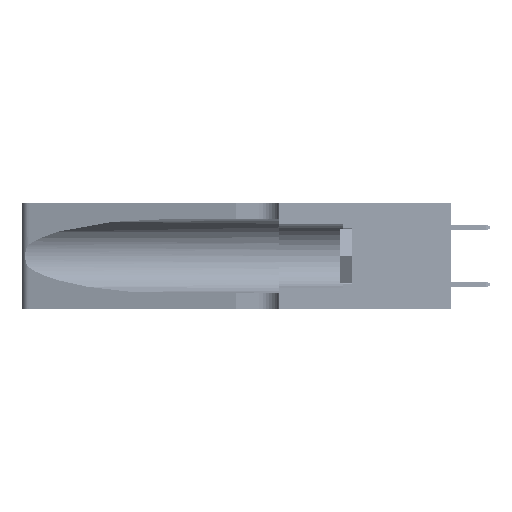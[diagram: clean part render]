
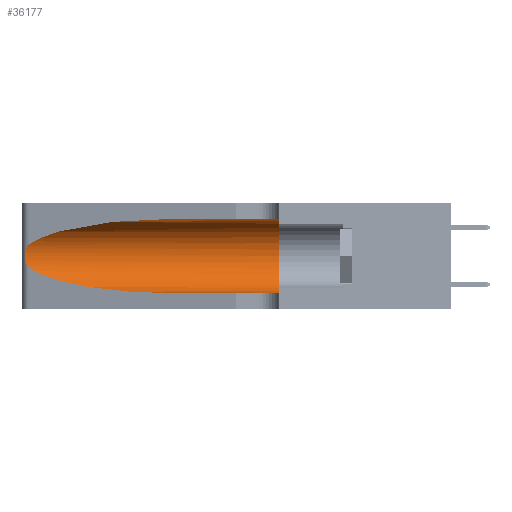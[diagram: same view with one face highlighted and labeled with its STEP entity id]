
A CAD part, left-side view. The second image highlights one B-rep face of the part: STEP entity #36177.
In plain terms, the highlighted cylindrical face has radius 3.308 mm (diameter 6.617 mm), a partial arc.
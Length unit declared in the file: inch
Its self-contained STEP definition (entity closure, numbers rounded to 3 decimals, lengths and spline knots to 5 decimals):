
#191 = VECTOR ( 'NONE', #29480, 39.37008 ) ;
#1337 = ORIENTED_EDGE ( 'NONE', *, *, #4520, .T. ) ;
#3465 = ORIENTED_EDGE ( 'NONE', *, *, #43835, .F. ) ;
#3618 = DIRECTION ( 'NONE',  ( 0., -1., 0. ) ) ;
#4151 = CARTESIAN_POINT ( 'NONE',  ( 0.25854, 1.2359, 0.20912 ) ) ;
#4520 = EDGE_CURVE ( 'NONE', #49002, #5500, #7059, .T. ) ;
#4654 = CARTESIAN_POINT ( 'NONE',  ( 0.25487, 1.22718, 0.22369 ) ) ;
#5500 = VERTEX_POINT ( 'NONE', #46580 ) ;
#6939 = CARTESIAN_POINT ( 'NONE',  ( 0.25555, 1.22994, 0.2215 ) ) ;
#7038 = VERTEX_POINT ( 'NONE', #29542 ) ;
#7059 = B_SPLINE_CURVE_WITH_KNOTS ( 'NONE', 3,
 ( #38008, #6939, #23204, #18938, #4151, #26720, #15172, #26460, #30473, #42260, #7921, #11437, #42010, #7432 ),
 .UNSPECIFIED., .F., .F.,
 ( 4, 2, 2, 2, 2, 2, 4 ),
 ( 0., 0.00027, 0.00053, 0.00107, 0.0016, 0.00187, 0.00214 ),
 .UNSPECIFIED. ) ;
#7432 = CARTESIAN_POINT ( 'NONE',  ( 0.25487, 1.22718, 0.14631 ) ) ;
#7582 = FACE_OUTER_BOUND ( 'NONE', #7714, .T. ) ;
#7714 = EDGE_LOOP ( 'NONE', ( #15590, #1337, #43993, #9065, #46394, #3465 ) ) ;
#7921 = CARTESIAN_POINT ( 'NONE',  ( 0.25789, 1.23486, 0.15765 ) ) ;
#8184 = CARTESIAN_POINT ( 'NONE',  ( 0.1305, 0.72297, 0.31525 ) ) ;
#9062 = CARTESIAN_POINT ( 'NONE',  ( 0.1305, 1.61858, 0.185 ) ) ;
#9065 = ORIENTED_EDGE ( 'NONE', *, *, #48445, .T. ) ;
#10133 = CIRCLE ( 'NONE', #30968, 0.13025 ) ;
#10639 = LINE ( 'NONE', #29927, #42033 ) ;
#11437 = CARTESIAN_POINT ( 'NONE',  ( 0.25639, 1.23186, 0.15144 ) ) ;
#15172 = CARTESIAN_POINT ( 'NONE',  ( 0.26075, 1.23896, 0.19203 ) ) ;
#15590 = ORIENTED_EDGE ( 'NONE', *, *, #33847, .T. ) ;
#18763 = CARTESIAN_POINT ( 'NONE',  ( 0.25487, 1.22718, 0.14631 ) ) ;
#18938 = CARTESIAN_POINT ( 'NONE',  ( 0.25787, 1.23484, 0.2124 ) ) ;
#19175 =( BOUNDED_CURVE ( )  B_SPLINE_CURVE ( 3, ( #8184, #23458, #41339, #4654 ),
 .UNSPECIFIED., .F., .T. ) 
 B_SPLINE_CURVE_WITH_KNOTS ( ( 4, 4 ),
 ( 1.5708, 2.84003 ),
 .UNSPECIFIED. ) 
 CURVE ( )  GEOMETRIC_REPRESENTATION_ITEM ( )  RATIONAL_B_SPLINE_CURVE ( ( 1., 0.87, 0.87, 1. ) ) 
 REPRESENTATION_ITEM ( '' )  );
#19764 = CARTESIAN_POINT ( 'NONE',  ( 0.1305, 0.72297, 0.05475 ) ) ;
#19955 = DIRECTION ( 'NONE',  ( 0., 1., 0. ) ) ;
#20069 = CYLINDRICAL_SURFACE ( 'NONE', #26952, 0.13025 ) ;
#20295 = VERTEX_POINT ( 'NONE', #32686 ) ;
#22842 = EDGE_CURVE ( 'NONE', #7038, #20295, #10133, .T. ) ;
#23204 = CARTESIAN_POINT ( 'NONE',  ( 0.25639, 1.23184, 0.21858 ) ) ;
#23458 = CARTESIAN_POINT ( 'NONE',  ( 0.18966, 0.96281, 0.31525 ) ) ;
#24816 = DIRECTION ( 'NONE',  ( 0., 0., -1. ) ) ;
#25413 = VERTEX_POINT ( 'NONE', #19764 ) ;
#26460 = CARTESIAN_POINT ( 'NONE',  ( 0.26075, 1.23896, 0.178 ) ) ;
#26720 = CARTESIAN_POINT ( 'NONE',  ( 0.26018, 1.23835, 0.19895 ) ) ;
#26952 = AXIS2_PLACEMENT_3D ( 'NONE', #9062, #31623, #24816 ) ;
#29480 = DIRECTION ( 'NONE',  ( 0., -1., 0. ) ) ;
#29542 = CARTESIAN_POINT ( 'NONE',  ( 0.1305, 0.35, 0.31525 ) ) ;
#29927 = CARTESIAN_POINT ( 'NONE',  ( 0.1305, 1.61858, 0.05475 ) ) ;
#30047 = EDGE_CURVE ( 'NONE', #5500, #25413, #39978, .T. ) ;
#30473 = CARTESIAN_POINT ( 'NONE',  ( 0.26017, 1.23833, 0.17102 ) ) ;
#30807 = CARTESIAN_POINT ( 'NONE',  ( 0.1305, 0.72297, 0.31525 ) ) ;
#30968 = AXIS2_PLACEMENT_3D ( 'NONE', #38793, #19955, #35257 ) ;
#31623 = DIRECTION ( 'NONE',  ( 0., -1., 0. ) ) ;
#32008 = CARTESIAN_POINT ( 'NONE',  ( 0.1305, 0.72297, 0.05475 ) ) ;
#32686 = CARTESIAN_POINT ( 'NONE',  ( 0.1305, 0.35, 0.05475 ) ) ;
#32988 = LINE ( 'NONE', #37004, #191 ) ;
#33847 = EDGE_CURVE ( 'NONE', #38002, #49002, #19175, .T. ) ;
#34073 = CARTESIAN_POINT ( 'NONE',  ( 0.2373, 1.15595, 0.08982 ) ) ;
#35257 = DIRECTION ( 'NONE',  ( 0., 0., 1. ) ) ;
#36177 = ADVANCED_FACE ( 'NONE', ( #7582 ), #20069, .F. ) ;
#37004 = CARTESIAN_POINT ( 'NONE',  ( 0.1305, 1.61858, 0.31525 ) ) ;
#38002 = VERTEX_POINT ( 'NONE', #30807 ) ;
#38008 = CARTESIAN_POINT ( 'NONE',  ( 0.25487, 1.22718, 0.22369 ) ) ;
#38793 = CARTESIAN_POINT ( 'NONE',  ( 0.1305, 0.35, 0.185 ) ) ;
#38829 = CARTESIAN_POINT ( 'NONE',  ( 0.18966, 0.96281, 0.05475 ) ) ;
#39978 =( BOUNDED_CURVE ( )  B_SPLINE_CURVE ( 3, ( #18763, #34073, #38829, #32008 ),
 .UNSPECIFIED., .F., .T. ) 
 B_SPLINE_CURVE_WITH_KNOTS ( ( 4, 4 ),
 ( 3.44316, 4.71239 ),
 .UNSPECIFIED. ) 
 CURVE ( )  GEOMETRIC_REPRESENTATION_ITEM ( )  RATIONAL_B_SPLINE_CURVE ( ( 1., 0.87, 0.87, 1. ) ) 
 REPRESENTATION_ITEM ( '' )  );
#41339 = CARTESIAN_POINT ( 'NONE',  ( 0.2373, 1.15595, 0.28018 ) ) ;
#41832 = CARTESIAN_POINT ( 'NONE',  ( 0.25487, 1.22718, 0.22369 ) ) ;
#42010 = CARTESIAN_POINT ( 'NONE',  ( 0.25555, 1.22993, 0.14849 ) ) ;
#42033 = VECTOR ( 'NONE', #3618, 39.37008 ) ;
#42260 = CARTESIAN_POINT ( 'NONE',  ( 0.25856, 1.23593, 0.16098 ) ) ;
#43835 = EDGE_CURVE ( 'NONE', #38002, #7038, #32988, .T. ) ;
#43993 = ORIENTED_EDGE ( 'NONE', *, *, #30047, .T. ) ;
#46394 = ORIENTED_EDGE ( 'NONE', *, *, #22842, .F. ) ;
#46580 = CARTESIAN_POINT ( 'NONE',  ( 0.25487, 1.22718, 0.14631 ) ) ;
#48445 = EDGE_CURVE ( 'NONE', #25413, #20295, #10639, .T. ) ;
#49002 = VERTEX_POINT ( 'NONE', #41832 ) ;
